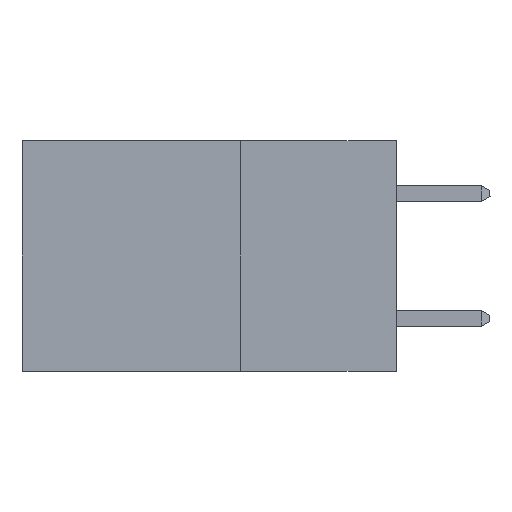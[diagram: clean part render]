
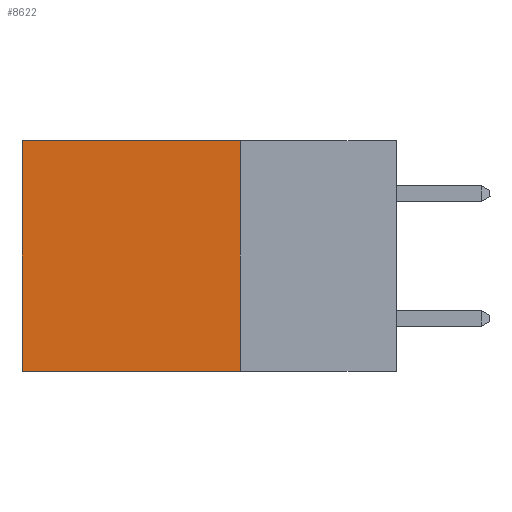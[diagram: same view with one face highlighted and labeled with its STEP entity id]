
A CAD part, left-side view. The second image highlights one B-rep face of the part: STEP entity #8622.
In plain terms, the highlighted planar face has unit normal (-1, 0, 0).
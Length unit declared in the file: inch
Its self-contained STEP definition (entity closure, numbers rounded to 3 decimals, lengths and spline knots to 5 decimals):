
#340 = VERTEX_POINT ( 'NONE', #4713 ) ;
#444 = DIRECTION ( 'NONE',  ( 0., 0., -1. ) ) ;
#2187 = VERTEX_POINT ( 'NONE', #9412 ) ;
#2329 = ORIENTED_EDGE ( 'NONE', *, *, #10051, .F. ) ;
#4017 = VECTOR ( 'NONE', #12845, 39.37008 ) ;
#4306 = VECTOR ( 'NONE', #444, 39.37008 ) ;
#4615 = EDGE_CURVE ( 'NONE', #9946, #2187, #11898, .T. ) ;
#4660 = CARTESIAN_POINT ( 'NONE',  ( 0.298, 0.25, 0. ) ) ;
#4713 = CARTESIAN_POINT ( 'NONE',  ( 0.298, 0.25, 0. ) ) ;
#5167 = VECTOR ( 'NONE', #11554, 39.37008 ) ;
#5651 = LINE ( 'NONE', #10725, #5167 ) ;
#5703 = VERTEX_POINT ( 'NONE', #8481 ) ;
#5848 = AXIS2_PLACEMENT_3D ( 'NONE', #4660, #10811, #11836 ) ;
#6824 = CARTESIAN_POINT ( 'NONE',  ( 0.298, 0.6, 0. ) ) ;
#7125 = ORIENTED_EDGE ( 'NONE', *, *, #12380, .T. ) ;
#7558 = EDGE_LOOP ( 'NONE', ( #11124, #2329, #10465, #7125 ) ) ;
#8144 = CARTESIAN_POINT ( 'NONE',  ( 0.298, 0.25, 0. ) ) ;
#8161 = LINE ( 'NONE', #11747, #4017 ) ;
#8481 = CARTESIAN_POINT ( 'NONE',  ( 0.298, 0.25, -0.37 ) ) ;
#8622 = ADVANCED_FACE ( 'NONE', ( #11126 ), #9814, .F. ) ;
#9412 = CARTESIAN_POINT ( 'NONE',  ( 0.298, 0.6, -0.37 ) ) ;
#9814 = PLANE ( 'NONE',  #5848 ) ;
#9908 = EDGE_CURVE ( 'NONE', #340, #5703, #8161, .T. ) ;
#9946 = VERTEX_POINT ( 'NONE', #13408 ) ;
#10051 = EDGE_CURVE ( 'NONE', #5703, #2187, #5651, .T. ) ;
#10465 = ORIENTED_EDGE ( 'NONE', *, *, #9908, .F. ) ;
#10725 = CARTESIAN_POINT ( 'NONE',  ( 0.298, 0.25, -0.37 ) ) ;
#10811 = DIRECTION ( 'NONE',  ( 1., 0., 0. ) ) ;
#11124 = ORIENTED_EDGE ( 'NONE', *, *, #4615, .T. ) ;
#11126 = FACE_OUTER_BOUND ( 'NONE', #7558, .T. ) ;
#11355 = VECTOR ( 'NONE', #12369, 39.37008 ) ;
#11554 = DIRECTION ( 'NONE',  ( 0., 1., 0. ) ) ;
#11747 = CARTESIAN_POINT ( 'NONE',  ( 0.298, 0.25, 0. ) ) ;
#11836 = DIRECTION ( 'NONE',  ( 0., 0., -1. ) ) ;
#11898 = LINE ( 'NONE', #6824, #4306 ) ;
#12352 = LINE ( 'NONE', #8144, #11355 ) ;
#12369 = DIRECTION ( 'NONE',  ( 0., 1., 0. ) ) ;
#12380 = EDGE_CURVE ( 'NONE', #340, #9946, #12352, .T. ) ;
#12845 = DIRECTION ( 'NONE',  ( 0., 0., -1. ) ) ;
#13408 = CARTESIAN_POINT ( 'NONE',  ( 0.298, 0.6, 0. ) ) ;
